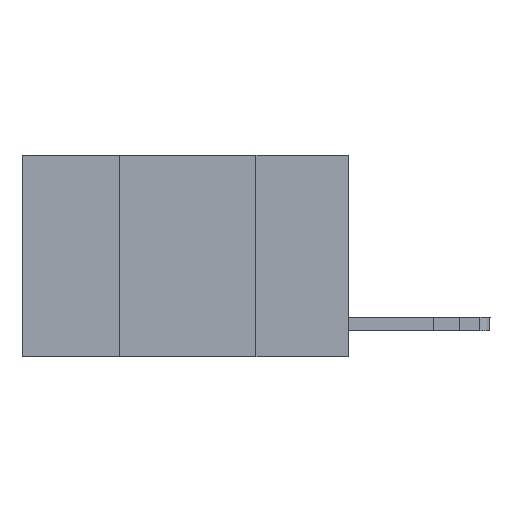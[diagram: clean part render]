
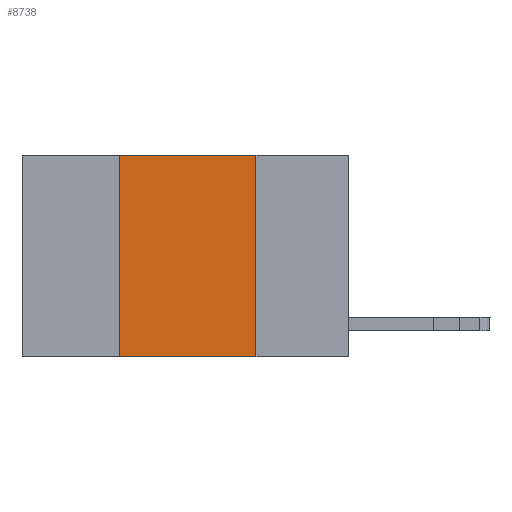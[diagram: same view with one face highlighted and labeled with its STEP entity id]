
A CAD part, left-side view. The second image highlights one B-rep face of the part: STEP entity #8738.
In plain terms, the highlighted planar face has unit normal (-1, 0, 0).
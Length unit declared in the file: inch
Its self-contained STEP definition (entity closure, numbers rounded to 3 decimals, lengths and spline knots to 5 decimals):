
#973 = CARTESIAN_POINT ( 'NONE',  ( 0., 0.42, 0. ) ) ;
#1306 = PLANE ( 'NONE',  #11334 ) ;
#1950 = LINE ( 'NONE', #4634, #12179 ) ;
#2295 = ORIENTED_EDGE ( 'NONE', *, *, #2560, .F. ) ;
#2410 = FACE_OUTER_BOUND ( 'NONE', #12998, .T. ) ;
#2552 = VERTEX_POINT ( 'NONE', #13478 ) ;
#2560 = EDGE_CURVE ( 'NONE', #2552, #15083, #15249, .T. ) ;
#2770 = CARTESIAN_POINT ( 'NONE',  ( 0., 0.17, 0. ) ) ;
#2827 = DIRECTION ( 'NONE',  ( 0., 0., -1. ) ) ;
#3829 = LINE ( 'NONE', #2770, #13505 ) ;
#4011 = DIRECTION ( 'NONE',  ( 0., 0., -1. ) ) ;
#4634 = CARTESIAN_POINT ( 'NONE',  ( 0., 0.6, 0. ) ) ;
#4684 = CARTESIAN_POINT ( 'NONE',  ( 0., 0.17, -0.37 ) ) ;
#4764 = ORIENTED_EDGE ( 'NONE', *, *, #6915, .T. ) ;
#4791 = EDGE_CURVE ( 'NONE', #15083, #8264, #1950, .T. ) ;
#5371 = VERTEX_POINT ( 'NONE', #4684 ) ;
#5763 = EDGE_CURVE ( 'NONE', #8264, #5371, #3829, .T. ) ;
#6093 = ORIENTED_EDGE ( 'NONE', *, *, #4791, .F. ) ;
#6915 = EDGE_CURVE ( 'NONE', #2552, #5371, #14020, .T. ) ;
#7412 = VECTOR ( 'NONE', #8792, 39.37008 ) ;
#7502 = CARTESIAN_POINT ( 'NONE',  ( 0., 0.6, -0.37 ) ) ;
#8264 = VERTEX_POINT ( 'NONE', #15674 ) ;
#8738 = ADVANCED_FACE ( 'NONE', ( #2410 ), #1306, .F. ) ;
#8792 = DIRECTION ( 'NONE',  ( 0., -1., 0. ) ) ;
#10371 = CARTESIAN_POINT ( 'NONE',  ( 0., 0.6, 0. ) ) ;
#11334 = AXIS2_PLACEMENT_3D ( 'NONE', #10371, #11611, #4011 ) ;
#11611 = DIRECTION ( 'NONE',  ( 1., 0., 0. ) ) ;
#12179 = VECTOR ( 'NONE', #12200, 39.37008 ) ;
#12200 = DIRECTION ( 'NONE',  ( 0., -1., 0. ) ) ;
#12825 = VECTOR ( 'NONE', #13204, 39.37008 ) ;
#12998 = EDGE_LOOP ( 'NONE', ( #13030, #6093, #2295, #4764 ) ) ;
#13030 = ORIENTED_EDGE ( 'NONE', *, *, #5763, .F. ) ;
#13204 = DIRECTION ( 'NONE',  ( 0., 0., 1. ) ) ;
#13224 = CARTESIAN_POINT ( 'NONE',  ( 0., 0.42, 0. ) ) ;
#13478 = CARTESIAN_POINT ( 'NONE',  ( 0., 0.42, -0.37 ) ) ;
#13505 = VECTOR ( 'NONE', #2827, 39.37008 ) ;
#14020 = LINE ( 'NONE', #7502, #7412 ) ;
#15083 = VERTEX_POINT ( 'NONE', #973 ) ;
#15249 = LINE ( 'NONE', #13224, #12825 ) ;
#15674 = CARTESIAN_POINT ( 'NONE',  ( 0., 0.17, 0. ) ) ;
